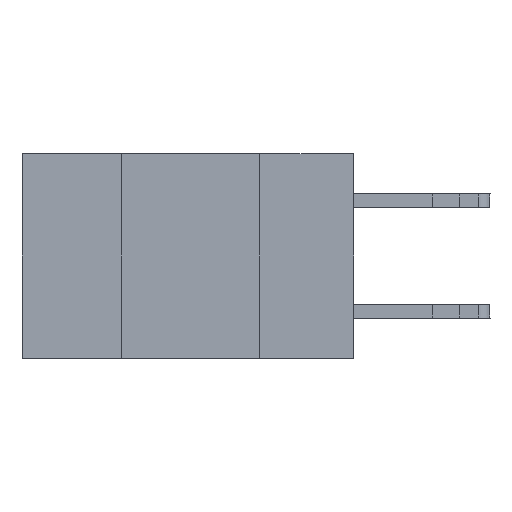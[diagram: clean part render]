
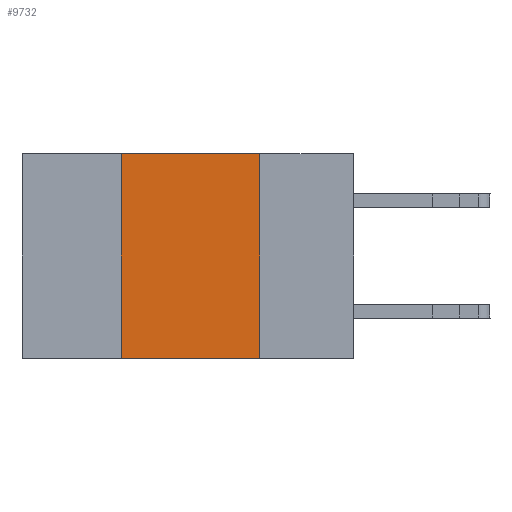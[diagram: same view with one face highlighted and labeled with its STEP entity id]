
A CAD part, left-side view. The second image highlights one B-rep face of the part: STEP entity #9732.
In plain terms, the highlighted planar face has unit normal (-1, 0, 0).
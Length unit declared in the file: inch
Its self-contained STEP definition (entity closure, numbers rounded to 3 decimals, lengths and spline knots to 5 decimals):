
#272 = EDGE_CURVE ( 'NONE', #16083, #18227, #19263, .T. ) ;
#482 = ORIENTED_EDGE ( 'NONE', *, *, #10772, .T. ) ;
#969 = ORIENTED_EDGE ( 'NONE', *, *, #272, .F. ) ;
#1764 = DIRECTION ( 'NONE',  ( 0., -1., 0. ) ) ;
#2204 = DIRECTION ( 'NONE',  ( 0., 0., 1. ) ) ;
#2587 = PLANE ( 'NONE',  #25214 ) ;
#4016 = CARTESIAN_POINT ( 'NONE',  ( 0., 0.42, 0. ) ) ;
#4723 = VECTOR ( 'NONE', #7994, 39.37008 ) ;
#4848 = CARTESIAN_POINT ( 'NONE',  ( 0., 0.17, 0. ) ) ;
#5643 = DIRECTION ( 'NONE',  ( 0., -1., 0. ) ) ;
#6370 = EDGE_LOOP ( 'NONE', ( #10672, #969, #14136, #482 ) ) ;
#7048 = VECTOR ( 'NONE', #1764, 39.37008 ) ;
#7163 = LINE ( 'NONE', #8244, #11378 ) ;
#7994 = DIRECTION ( 'NONE',  ( 0., 0., -1. ) ) ;
#8244 = CARTESIAN_POINT ( 'NONE',  ( 0., 0.42, 0. ) ) ;
#9581 = CARTESIAN_POINT ( 'NONE',  ( 0., 0.17, -0.37 ) ) ;
#9732 = ADVANCED_FACE ( 'NONE', ( #32488 ), #2587, .F. ) ;
#10672 = ORIENTED_EDGE ( 'NONE', *, *, #32664, .F. ) ;
#10772 = EDGE_CURVE ( 'NONE', #19344, #22548, #21119, .T. ) ;
#10849 = CARTESIAN_POINT ( 'NONE',  ( 0., 0.42, -0.37 ) ) ;
#11378 = VECTOR ( 'NONE', #2204, 39.37008 ) ;
#12592 = EDGE_CURVE ( 'NONE', #19344, #16083, #7163, .T. ) ;
#14136 = ORIENTED_EDGE ( 'NONE', *, *, #12592, .F. ) ;
#14263 = DIRECTION ( 'NONE',  ( 0., 0., -1. ) ) ;
#16083 = VERTEX_POINT ( 'NONE', #4016 ) ;
#16689 = CARTESIAN_POINT ( 'NONE',  ( 0., 0.17, 0. ) ) ;
#18227 = VERTEX_POINT ( 'NONE', #16689 ) ;
#19263 = LINE ( 'NONE', #31978, #7048 ) ;
#19344 = VERTEX_POINT ( 'NONE', #10849 ) ;
#21119 = LINE ( 'NONE', #29948, #36191 ) ;
#22548 = VERTEX_POINT ( 'NONE', #9581 ) ;
#25214 = AXIS2_PLACEMENT_3D ( 'NONE', #26491, #38187, #14263 ) ;
#26491 = CARTESIAN_POINT ( 'NONE',  ( 0., 0.6, 0. ) ) ;
#29948 = CARTESIAN_POINT ( 'NONE',  ( 0., 0.6, -0.37 ) ) ;
#31978 = CARTESIAN_POINT ( 'NONE',  ( 0., 0.6, 0. ) ) ;
#32488 = FACE_OUTER_BOUND ( 'NONE', #6370, .T. ) ;
#32664 = EDGE_CURVE ( 'NONE', #18227, #22548, #36693, .T. ) ;
#36191 = VECTOR ( 'NONE', #5643, 39.37008 ) ;
#36693 = LINE ( 'NONE', #4848, #4723 ) ;
#38187 = DIRECTION ( 'NONE',  ( 1., 0., 0. ) ) ;
